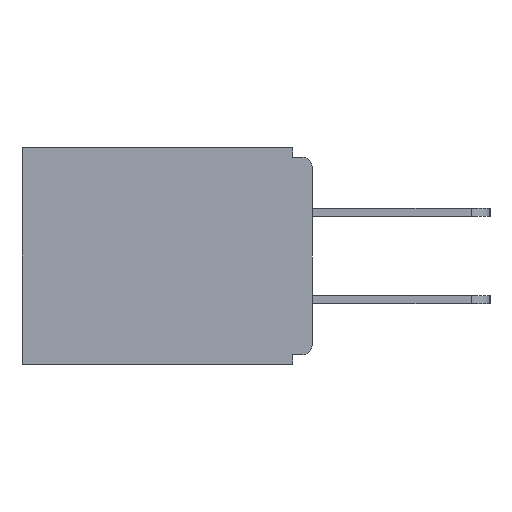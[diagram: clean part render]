
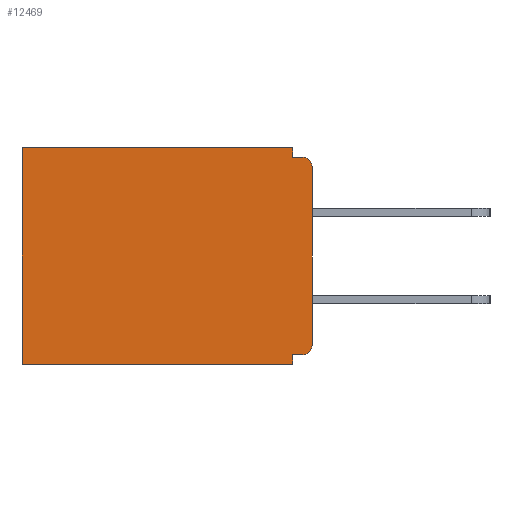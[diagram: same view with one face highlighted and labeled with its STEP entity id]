
A CAD part, left-side view. The second image highlights one B-rep face of the part: STEP entity #12469.
In plain terms, the highlighted planar face has unit normal (-1, 0, 0).
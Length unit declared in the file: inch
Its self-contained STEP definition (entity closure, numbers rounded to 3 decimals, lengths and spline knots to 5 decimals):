
#77 = EDGE_CURVE ( 'NONE', #12377, #11269, #18210, .T. ) ;
#165 = DIRECTION ( 'NONE',  ( 0., 0., -1. ) ) ;
#491 = CARTESIAN_POINT ( 'NONE',  ( 0.298, 0.031, -0.328 ) ) ;
#493 = LINE ( 'NONE', #5717, #3603 ) ;
#1059 = CARTESIAN_POINT ( 'NONE',  ( 0.298, 0.015, -0.03 ) ) ;
#1174 = EDGE_CURVE ( 'NONE', #7061, #17833, #493, .T. ) ;
#1330 = DIRECTION ( 'NONE',  ( 0., 1., 0. ) ) ;
#1891 = LINE ( 'NONE', #17982, #16889 ) ;
#1982 = CARTESIAN_POINT ( 'NONE',  ( 0.298, 0., 0. ) ) ;
#2471 = EDGE_CURVE ( 'NONE', #17833, #6144, #9082, .T. ) ;
#2748 = VECTOR ( 'NONE', #10805, 39.37008 ) ;
#3327 = CARTESIAN_POINT ( 'NONE',  ( 0.298, 0.015, -0.313 ) ) ;
#3603 = VECTOR ( 'NONE', #165, 39.37008 ) ;
#3666 = EDGE_CURVE ( 'NONE', #11712, #5539, #16972, .T. ) ;
#3868 = CARTESIAN_POINT ( 'NONE',  ( 0.298, 0.46, 0. ) ) ;
#4419 = ORIENTED_EDGE ( 'NONE', *, *, #17134, .T. ) ;
#4949 = CARTESIAN_POINT ( 'NONE',  ( 0.298, 0., -0.015 ) ) ;
#5128 = CARTESIAN_POINT ( 'NONE',  ( 0.298, 0., -0.313 ) ) ;
#5130 = LINE ( 'NONE', #7345, #14404 ) ;
#5337 = ORIENTED_EDGE ( 'NONE', *, *, #77, .T. ) ;
#5352 = LINE ( 'NONE', #12685, #12435 ) ;
#5539 = VERTEX_POINT ( 'NONE', #15699 ) ;
#5717 = CARTESIAN_POINT ( 'NONE',  ( 0.298, 0.031, -0.343 ) ) ;
#6029 = DIRECTION ( 'NONE',  ( -1., 0., 0. ) ) ;
#6144 = VERTEX_POINT ( 'NONE', #16207 ) ;
#6825 = CARTESIAN_POINT ( 'NONE',  ( 0.298, 0.031, -0.015 ) ) ;
#6838 = VERTEX_POINT ( 'NONE', #12114 ) ;
#6884 = VECTOR ( 'NONE', #17843, 39.37008 ) ;
#7019 = VECTOR ( 'NONE', #15805, 39.37008 ) ;
#7061 = VERTEX_POINT ( 'NONE', #13899 ) ;
#7345 = CARTESIAN_POINT ( 'NONE',  ( 0.298, 0., -0.343 ) ) ;
#7846 = ORIENTED_EDGE ( 'NONE', *, *, #16646, .F. ) ;
#7913 = EDGE_CURVE ( 'NONE', #6838, #10025, #9945, .T. ) ;
#7983 = VECTOR ( 'NONE', #9203, 39.37008 ) ;
#8146 = ORIENTED_EDGE ( 'NONE', *, *, #11432, .T. ) ;
#9082 = LINE ( 'NONE', #4949, #7983 ) ;
#9203 = DIRECTION ( 'NONE',  ( 0., -1., 0. ) ) ;
#9580 = DIRECTION ( 'NONE',  ( -1., 0., 0. ) ) ;
#9945 = CIRCLE ( 'NONE', #10084, 0.015 ) ;
#10025 = VERTEX_POINT ( 'NONE', #5128 ) ;
#10084 = AXIS2_PLACEMENT_3D ( 'NONE', #3327, #6029, #15927 ) ;
#10157 = CARTESIAN_POINT ( 'NONE',  ( 0.298, 0.46, -0.343 ) ) ;
#10414 = PLANE ( 'NONE',  #12956 ) ;
#10805 = DIRECTION ( 'NONE',  ( 0., 0., -1. ) ) ;
#10838 = ORIENTED_EDGE ( 'NONE', *, *, #1174, .F. ) ;
#11127 = DIRECTION ( 'NONE',  ( 1., 0., 0. ) ) ;
#11269 = VERTEX_POINT ( 'NONE', #10157 ) ;
#11432 = EDGE_CURVE ( 'NONE', #7061, #12377, #1891, .T. ) ;
#11496 = ORIENTED_EDGE ( 'NONE', *, *, #12599, .F. ) ;
#11641 = DIRECTION ( 'NONE',  ( 0., 1., 0. ) ) ;
#11712 = VERTEX_POINT ( 'NONE', #491 ) ;
#11974 = CIRCLE ( 'NONE', #16781, 0.015 ) ;
#12002 = FACE_OUTER_BOUND ( 'NONE', #17481, .T. ) ;
#12114 = CARTESIAN_POINT ( 'NONE',  ( 0.298, 0.015, -0.328 ) ) ;
#12377 = VERTEX_POINT ( 'NONE', #14080 ) ;
#12435 = VECTOR ( 'NONE', #1330, 39.37008 ) ;
#12469 = ADVANCED_FACE ( 'NONE', ( #12002 ), #10414, .F. ) ;
#12599 = EDGE_CURVE ( 'NONE', #13947, #10025, #15301, .T. ) ;
#12685 = CARTESIAN_POINT ( 'NONE',  ( 0.298, 0., -0.328 ) ) ;
#12956 = AXIS2_PLACEMENT_3D ( 'NONE', #1982, #11127, #16244 ) ;
#13098 = CARTESIAN_POINT ( 'NONE',  ( 0.298, 0., 0. ) ) ;
#13899 = CARTESIAN_POINT ( 'NONE',  ( 0.298, 0.031, 0. ) ) ;
#13926 = ORIENTED_EDGE ( 'NONE', *, *, #2471, .F. ) ;
#13947 = VERTEX_POINT ( 'NONE', #17204 ) ;
#14080 = CARTESIAN_POINT ( 'NONE',  ( 0.298, 0.46, 0. ) ) ;
#14404 = VECTOR ( 'NONE', #11641, 39.37008 ) ;
#15301 = LINE ( 'NONE', #13098, #6884 ) ;
#15339 = ORIENTED_EDGE ( 'NONE', *, *, #7913, .T. ) ;
#15699 = CARTESIAN_POINT ( 'NONE',  ( 0.298, 0.031, -0.343 ) ) ;
#15805 = DIRECTION ( 'NONE',  ( 0., 0., -1. ) ) ;
#15927 = DIRECTION ( 'NONE',  ( 0., 0., -1. ) ) ;
#16207 = CARTESIAN_POINT ( 'NONE',  ( 0.298, 0.015, -0.015 ) ) ;
#16244 = DIRECTION ( 'NONE',  ( 0., 0., -1. ) ) ;
#16646 = EDGE_CURVE ( 'NONE', #6838, #11712, #5352, .T. ) ;
#16680 = DIRECTION ( 'NONE',  ( 0., 0., -1. ) ) ;
#16772 = EDGE_CURVE ( 'NONE', #5539, #11269, #5130, .T. ) ;
#16781 = AXIS2_PLACEMENT_3D ( 'NONE', #1059, #9580, #16680 ) ;
#16889 = VECTOR ( 'NONE', #18044, 39.37008 ) ;
#16941 = ORIENTED_EDGE ( 'NONE', *, *, #16772, .F. ) ;
#16972 = LINE ( 'NONE', #17097, #7019 ) ;
#17097 = CARTESIAN_POINT ( 'NONE',  ( 0.298, 0.031, -0.343 ) ) ;
#17134 = EDGE_CURVE ( 'NONE', #13947, #6144, #11974, .T. ) ;
#17204 = CARTESIAN_POINT ( 'NONE',  ( 0.298, 0., -0.03 ) ) ;
#17338 = ORIENTED_EDGE ( 'NONE', *, *, #3666, .F. ) ;
#17481 = EDGE_LOOP ( 'NONE', ( #4419, #13926, #10838, #8146, #5337, #16941, #17338, #7846, #15339, #11496 ) ) ;
#17833 = VERTEX_POINT ( 'NONE', #6825 ) ;
#17843 = DIRECTION ( 'NONE',  ( 0., 0., -1. ) ) ;
#17982 = CARTESIAN_POINT ( 'NONE',  ( 0.298, 0., 0. ) ) ;
#18044 = DIRECTION ( 'NONE',  ( 0., 1., 0. ) ) ;
#18210 = LINE ( 'NONE', #3868, #2748 ) ;
